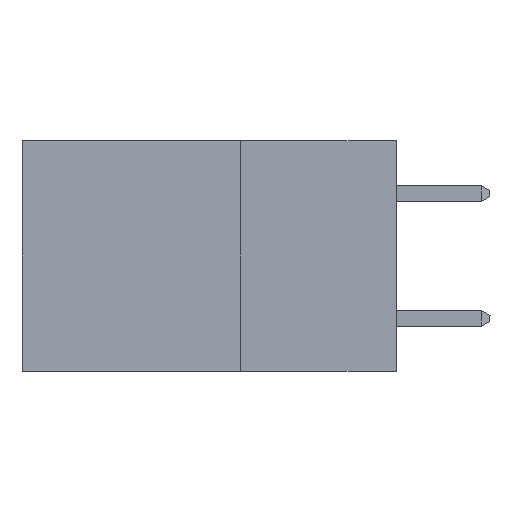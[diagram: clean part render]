
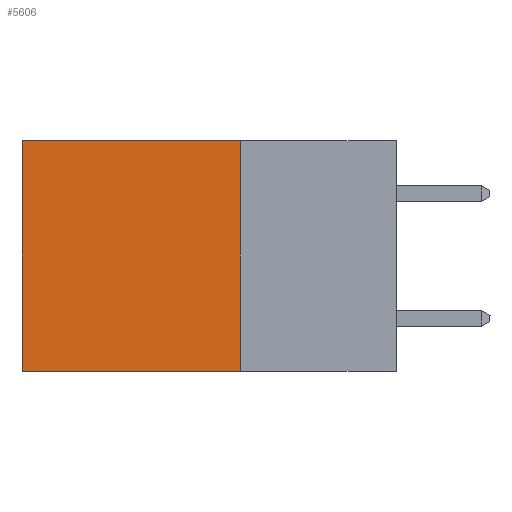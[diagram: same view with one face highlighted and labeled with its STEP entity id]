
A CAD part, left-side view. The second image highlights one B-rep face of the part: STEP entity #5606.
In plain terms, the highlighted planar face has unit normal (-1, 0, 0).
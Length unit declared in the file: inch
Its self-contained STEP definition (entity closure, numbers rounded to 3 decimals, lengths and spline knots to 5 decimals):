
#570 = VECTOR ( 'NONE', #9624, 39.37008 ) ;
#1196 = VERTEX_POINT ( 'NONE', #7704 ) ;
#1316 = CARTESIAN_POINT ( 'NONE',  ( 0.298, 0.25, 0. ) ) ;
#1356 = CARTESIAN_POINT ( 'NONE',  ( 0.298, 0.25, -0.37 ) ) ;
#1583 = CARTESIAN_POINT ( 'NONE',  ( 0.298, 0.6, 0. ) ) ;
#1960 = CARTESIAN_POINT ( 'NONE',  ( 0.298, 0.25, 0. ) ) ;
#2235 = EDGE_CURVE ( 'NONE', #7538, #7051, #9816, .T. ) ;
#2421 = EDGE_LOOP ( 'NONE', ( #3970, #3853, #4488, #8281 ) ) ;
#2531 = DIRECTION ( 'NONE',  ( 0., 0., -1. ) ) ;
#2603 = CARTESIAN_POINT ( 'NONE',  ( 0.298, 0.25, 0. ) ) ;
#3853 = ORIENTED_EDGE ( 'NONE', *, *, #6899, .F. ) ;
#3970 = ORIENTED_EDGE ( 'NONE', *, *, #4794, .T. ) ;
#3986 = VECTOR ( 'NONE', #2531, 39.37008 ) ;
#4324 = LINE ( 'NONE', #5940, #9770 ) ;
#4486 = VECTOR ( 'NONE', #4873, 39.37008 ) ;
#4488 = ORIENTED_EDGE ( 'NONE', *, *, #8344, .F. ) ;
#4794 = EDGE_CURVE ( 'NONE', #7051, #1196, #10168, .T. ) ;
#4873 = DIRECTION ( 'NONE',  ( 0., 1., 0. ) ) ;
#5295 = DIRECTION ( 'NONE',  ( 1., 0., 0. ) ) ;
#5606 = ADVANCED_FACE ( 'NONE', ( #9144 ), #7045, .F. ) ;
#5829 = CARTESIAN_POINT ( 'NONE',  ( 0.298, 0.6, 0. ) ) ;
#5940 = CARTESIAN_POINT ( 'NONE',  ( 0.298, 0.25, 0. ) ) ;
#6247 = AXIS2_PLACEMENT_3D ( 'NONE', #2603, #5295, #7001 ) ;
#6899 = EDGE_CURVE ( 'NONE', #9146, #1196, #7324, .T. ) ;
#7001 = DIRECTION ( 'NONE',  ( 0., 0., -1. ) ) ;
#7045 = PLANE ( 'NONE',  #6247 ) ;
#7051 = VERTEX_POINT ( 'NONE', #5829 ) ;
#7071 = CARTESIAN_POINT ( 'NONE',  ( 0.298, 0.25, -0.37 ) ) ;
#7324 = LINE ( 'NONE', #1356, #570 ) ;
#7538 = VERTEX_POINT ( 'NONE', #1960 ) ;
#7704 = CARTESIAN_POINT ( 'NONE',  ( 0.298, 0.6, -0.37 ) ) ;
#8281 = ORIENTED_EDGE ( 'NONE', *, *, #2235, .T. ) ;
#8344 = EDGE_CURVE ( 'NONE', #7538, #9146, #4324, .T. ) ;
#9144 = FACE_OUTER_BOUND ( 'NONE', #2421, .T. ) ;
#9146 = VERTEX_POINT ( 'NONE', #7071 ) ;
#9624 = DIRECTION ( 'NONE',  ( 0., 1., 0. ) ) ;
#9770 = VECTOR ( 'NONE', #9801, 39.37008 ) ;
#9801 = DIRECTION ( 'NONE',  ( 0., 0., -1. ) ) ;
#9816 = LINE ( 'NONE', #1316, #4486 ) ;
#10168 = LINE ( 'NONE', #1583, #3986 ) ;
